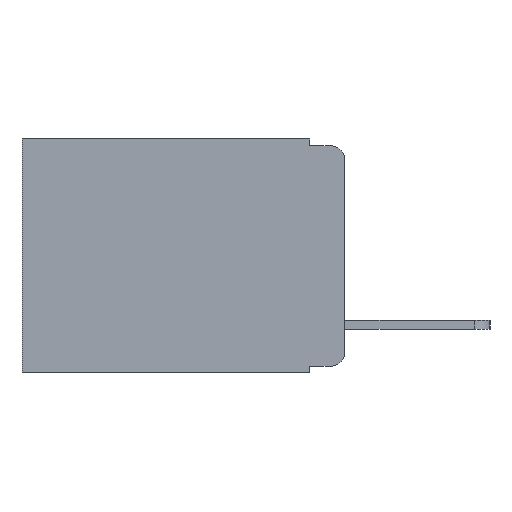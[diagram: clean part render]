
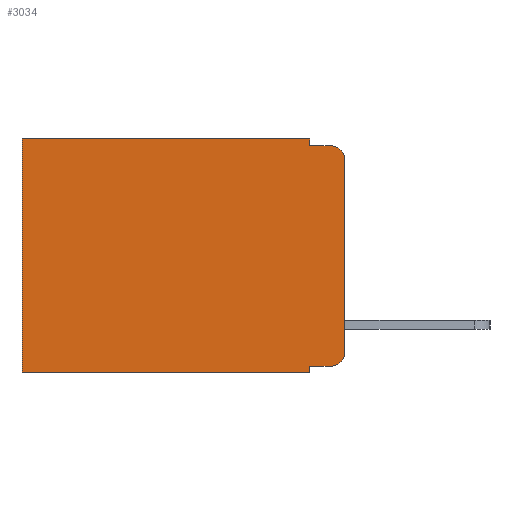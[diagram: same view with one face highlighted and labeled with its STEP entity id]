
A CAD part, left-side view. The second image highlights one B-rep face of the part: STEP entity #3034.
In plain terms, the highlighted planar face has unit normal (-1, 0, 0).
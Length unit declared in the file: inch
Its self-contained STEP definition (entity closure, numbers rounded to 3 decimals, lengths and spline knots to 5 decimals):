
#105 = CARTESIAN_POINT ( 'NONE',  ( 0.298, 0.02, -0.01 ) ) ;
#106 = DIRECTION ( 'NONE',  ( 0., 1., 0. ) ) ;
#285 = VERTEX_POINT ( 'NONE', #1430 ) ;
#342 = VERTEX_POINT ( 'NONE', #2901 ) ;
#372 = VECTOR ( 'NONE', #9901, 39.37008 ) ;
#823 = CARTESIAN_POINT ( 'NONE',  ( 0.298, 0., 0. ) ) ;
#1055 = LINE ( 'NONE', #1641, #10340 ) ;
#1103 = DIRECTION ( 'NONE',  ( 0., 1., 0. ) ) ;
#1273 = PLANE ( 'NONE',  #10067 ) ;
#1430 = CARTESIAN_POINT ( 'NONE',  ( 0.298, 0.473, -0.343 ) ) ;
#1450 = EDGE_CURVE ( 'NONE', #1918, #285, #1055, .T. ) ;
#1464 = DIRECTION ( 'NONE',  ( 0., 0., -1. ) ) ;
#1503 = FACE_OUTER_BOUND ( 'NONE', #3781, .T. ) ;
#1641 = CARTESIAN_POINT ( 'NONE',  ( 0.298, 0., -0.343 ) ) ;
#1815 = DIRECTION ( 'NONE',  ( 1., 0., 0. ) ) ;
#1869 = EDGE_CURVE ( 'NONE', #6390, #10360, #9499, .T. ) ;
#1918 = VERTEX_POINT ( 'NONE', #7741 ) ;
#2287 = ORIENTED_EDGE ( 'NONE', *, *, #7222, .T. ) ;
#2315 = CIRCLE ( 'NONE', #3796, 0.02 ) ;
#2427 = VECTOR ( 'NONE', #106, 39.37008 ) ;
#2568 = AXIS2_PLACEMENT_3D ( 'NONE', #11057, #11023, #10774 ) ;
#2901 = CARTESIAN_POINT ( 'NONE',  ( 0.298, 0.051, -0.333 ) ) ;
#3034 = ADVANCED_FACE ( 'NONE', ( #1503 ), #1273, .F. ) ;
#3210 = VERTEX_POINT ( 'NONE', #7517 ) ;
#3288 = DIRECTION ( 'NONE',  ( 0., -1., 0. ) ) ;
#3299 = CIRCLE ( 'NONE', #2568, 0.02 ) ;
#3447 = EDGE_CURVE ( 'NONE', #6390, #3210, #10298, .T. ) ;
#3452 = ORIENTED_EDGE ( 'NONE', *, *, #4772, .F. ) ;
#3617 = ORIENTED_EDGE ( 'NONE', *, *, #1450, .F. ) ;
#3781 = EDGE_LOOP ( 'NONE', ( #7778, #7914, #9205, #9785, #9643, #6947, #3617, #3452, #4248, #2287 ) ) ;
#3796 = AXIS2_PLACEMENT_3D ( 'NONE', #9004, #5232, #10242 ) ;
#3862 = EDGE_CURVE ( 'NONE', #5981, #4928, #3299, .T. ) ;
#4206 = DIRECTION ( 'NONE',  ( 0., 0., -1. ) ) ;
#4248 = ORIENTED_EDGE ( 'NONE', *, *, #6006, .T. ) ;
#4293 = CARTESIAN_POINT ( 'NONE',  ( 0.298, 0., 0. ) ) ;
#4346 = VERTEX_POINT ( 'NONE', #6914 ) ;
#4545 = LINE ( 'NONE', #8072, #11187 ) ;
#4558 = CARTESIAN_POINT ( 'NONE',  ( 0.298, 0.051, 0. ) ) ;
#4772 = EDGE_CURVE ( 'NONE', #342, #1918, #8439, .T. ) ;
#4928 = VERTEX_POINT ( 'NONE', #105 ) ;
#5232 = DIRECTION ( 'NONE',  ( -1., 0., 0. ) ) ;
#5565 = DIRECTION ( 'NONE',  ( 0., 0., -1. ) ) ;
#5817 = EDGE_CURVE ( 'NONE', #5981, #4346, #7013, .T. ) ;
#5872 = VECTOR ( 'NONE', #10000, 39.37008 ) ;
#5981 = VERTEX_POINT ( 'NONE', #10068 ) ;
#6006 = EDGE_CURVE ( 'NONE', #342, #8131, #9686, .T. ) ;
#6034 = VECTOR ( 'NONE', #5565, 39.37008 ) ;
#6161 = DIRECTION ( 'NONE',  ( 0., 0., -1. ) ) ;
#6390 = VERTEX_POINT ( 'NONE', #9893 ) ;
#6392 = EDGE_CURVE ( 'NONE', #3210, #4928, #8568, .T. ) ;
#6516 = CARTESIAN_POINT ( 'NONE',  ( 0.298, 0.02, -0.333 ) ) ;
#6808 = EDGE_CURVE ( 'NONE', #10360, #285, #4545, .T. ) ;
#6914 = CARTESIAN_POINT ( 'NONE',  ( 0.298, 0., -0.313 ) ) ;
#6947 = ORIENTED_EDGE ( 'NONE', *, *, #6808, .T. ) ;
#7013 = LINE ( 'NONE', #823, #9131 ) ;
#7101 = CARTESIAN_POINT ( 'NONE',  ( 0.298, 0.051, -0.333 ) ) ;
#7222 = EDGE_CURVE ( 'NONE', #8131, #4346, #2315, .T. ) ;
#7281 = VECTOR ( 'NONE', #3288, 39.37008 ) ;
#7517 = CARTESIAN_POINT ( 'NONE',  ( 0.298, 0.051, -0.01 ) ) ;
#7741 = CARTESIAN_POINT ( 'NONE',  ( 0.298, 0.051, -0.343 ) ) ;
#7778 = ORIENTED_EDGE ( 'NONE', *, *, #5817, .F. ) ;
#7914 = ORIENTED_EDGE ( 'NONE', *, *, #3862, .T. ) ;
#8072 = CARTESIAN_POINT ( 'NONE',  ( 0.298, 0.473, 0. ) ) ;
#8131 = VERTEX_POINT ( 'NONE', #6516 ) ;
#8439 = LINE ( 'NONE', #4558, #6034 ) ;
#8568 = LINE ( 'NONE', #9767, #5872 ) ;
#9004 = CARTESIAN_POINT ( 'NONE',  ( 0.298, 0.02, -0.313 ) ) ;
#9131 = VECTOR ( 'NONE', #6161, 39.37008 ) ;
#9205 = ORIENTED_EDGE ( 'NONE', *, *, #6392, .F. ) ;
#9499 = LINE ( 'NONE', #9749, #2427 ) ;
#9535 = CARTESIAN_POINT ( 'NONE',  ( 0.298, 0.473, 0. ) ) ;
#9643 = ORIENTED_EDGE ( 'NONE', *, *, #1869, .T. ) ;
#9686 = LINE ( 'NONE', #7101, #7281 ) ;
#9749 = CARTESIAN_POINT ( 'NONE',  ( 0.298, 0., 0. ) ) ;
#9767 = CARTESIAN_POINT ( 'NONE',  ( 0.298, 0.051, -0.01 ) ) ;
#9785 = ORIENTED_EDGE ( 'NONE', *, *, #3447, .F. ) ;
#9893 = CARTESIAN_POINT ( 'NONE',  ( 0.298, 0.051, 0. ) ) ;
#9901 = DIRECTION ( 'NONE',  ( 0., 0., -1. ) ) ;
#10000 = DIRECTION ( 'NONE',  ( 0., -1., 0. ) ) ;
#10067 = AXIS2_PLACEMENT_3D ( 'NONE', #4293, #1815, #1464 ) ;
#10068 = CARTESIAN_POINT ( 'NONE',  ( 0.298, 0., -0.03 ) ) ;
#10242 = DIRECTION ( 'NONE',  ( 0., 0., -1. ) ) ;
#10298 = LINE ( 'NONE', #10525, #372 ) ;
#10340 = VECTOR ( 'NONE', #1103, 39.37008 ) ;
#10360 = VERTEX_POINT ( 'NONE', #9535 ) ;
#10525 = CARTESIAN_POINT ( 'NONE',  ( 0.298, 0.051, 0. ) ) ;
#10774 = DIRECTION ( 'NONE',  ( 0., 0., -1. ) ) ;
#11023 = DIRECTION ( 'NONE',  ( -1., 0., 0. ) ) ;
#11057 = CARTESIAN_POINT ( 'NONE',  ( 0.298, 0.02, -0.03 ) ) ;
#11187 = VECTOR ( 'NONE', #4206, 39.37008 ) ;
